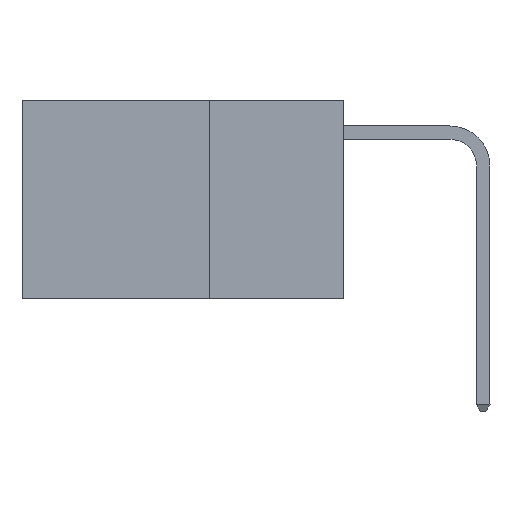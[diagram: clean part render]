
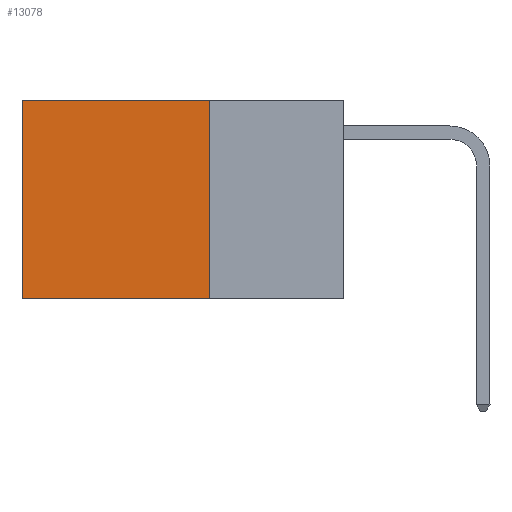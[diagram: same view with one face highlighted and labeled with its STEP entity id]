
A CAD part, left-side view. The second image highlights one B-rep face of the part: STEP entity #13078.
In plain terms, the highlighted planar face has unit normal (-1, 0, 0).
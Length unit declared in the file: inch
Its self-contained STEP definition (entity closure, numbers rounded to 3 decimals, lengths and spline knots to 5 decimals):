
#88 = CARTESIAN_POINT ( 'NONE',  ( 0.2625, 0.25, -0.37 ) ) ;
#242 = DIRECTION ( 'NONE',  ( 0., 0., -1. ) ) ;
#519 = CARTESIAN_POINT ( 'NONE',  ( 0.2625, 0.6, 0. ) ) ;
#1023 = ORIENTED_EDGE ( 'NONE', *, *, #14550, .T. ) ;
#1353 = CARTESIAN_POINT ( 'NONE',  ( 0.2625, 0.6, 0. ) ) ;
#1406 = AXIS2_PLACEMENT_3D ( 'NONE', #2601, #7219, #242 ) ;
#1445 = ORIENTED_EDGE ( 'NONE', *, *, #13027, .F. ) ;
#1522 = ORIENTED_EDGE ( 'NONE', *, *, #3798, .F. ) ;
#2136 = VERTEX_POINT ( 'NONE', #7993 ) ;
#2277 = ORIENTED_EDGE ( 'NONE', *, *, #9125, .T. ) ;
#2601 = CARTESIAN_POINT ( 'NONE',  ( 0.2625, 0.25, 0. ) ) ;
#2769 = EDGE_LOOP ( 'NONE', ( #2277, #1445, #1522, #1023 ) ) ;
#3798 = EDGE_CURVE ( 'NONE', #10768, #2136, #6249, .T. ) ;
#4010 = DIRECTION ( 'NONE',  ( 0., 0., -1. ) ) ;
#4113 = CARTESIAN_POINT ( 'NONE',  ( 0.2625, 0.6, -0.37 ) ) ;
#4350 = VERTEX_POINT ( 'NONE', #4113 ) ;
#6109 = LINE ( 'NONE', #519, #11940 ) ;
#6249 = LINE ( 'NONE', #11906, #8837 ) ;
#6717 = VECTOR ( 'NONE', #7107, 39.37008 ) ;
#7024 = CARTESIAN_POINT ( 'NONE',  ( 0.2625, 0.25, 0. ) ) ;
#7107 = DIRECTION ( 'NONE',  ( 0., 1., 0. ) ) ;
#7219 = DIRECTION ( 'NONE',  ( 1., 0., 0. ) ) ;
#7234 = CARTESIAN_POINT ( 'NONE',  ( 0.2625, 0.25, 0. ) ) ;
#7650 = DIRECTION ( 'NONE',  ( 0., 0., -1. ) ) ;
#7993 = CARTESIAN_POINT ( 'NONE',  ( 0.2625, 0.25, -0.37 ) ) ;
#8073 = LINE ( 'NONE', #7234, #10926 ) ;
#8837 = VECTOR ( 'NONE', #7650, 39.37008 ) ;
#9125 = EDGE_CURVE ( 'NONE', #9567, #4350, #6109, .T. ) ;
#9567 = VERTEX_POINT ( 'NONE', #1353 ) ;
#9606 = LINE ( 'NONE', #88, #6717 ) ;
#10768 = VERTEX_POINT ( 'NONE', #7024 ) ;
#10926 = VECTOR ( 'NONE', #12673, 39.37008 ) ;
#11906 = CARTESIAN_POINT ( 'NONE',  ( 0.2625, 0.25, 0. ) ) ;
#11940 = VECTOR ( 'NONE', #4010, 39.37008 ) ;
#12673 = DIRECTION ( 'NONE',  ( 0., 1., 0. ) ) ;
#13027 = EDGE_CURVE ( 'NONE', #2136, #4350, #9606, .T. ) ;
#13078 = ADVANCED_FACE ( 'NONE', ( #14393 ), #13740, .F. ) ;
#13740 = PLANE ( 'NONE',  #1406 ) ;
#14393 = FACE_OUTER_BOUND ( 'NONE', #2769, .T. ) ;
#14550 = EDGE_CURVE ( 'NONE', #10768, #9567, #8073, .T. ) ;
